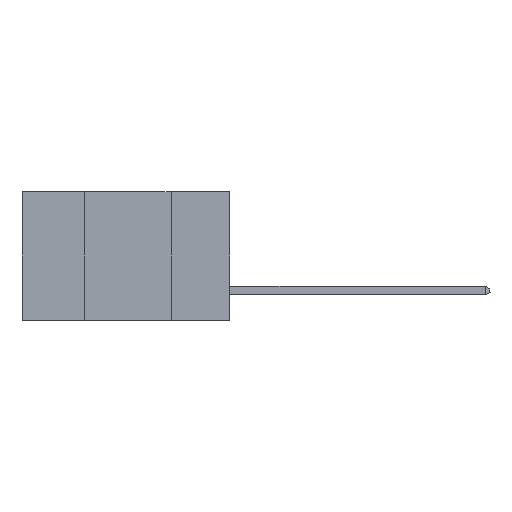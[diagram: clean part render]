
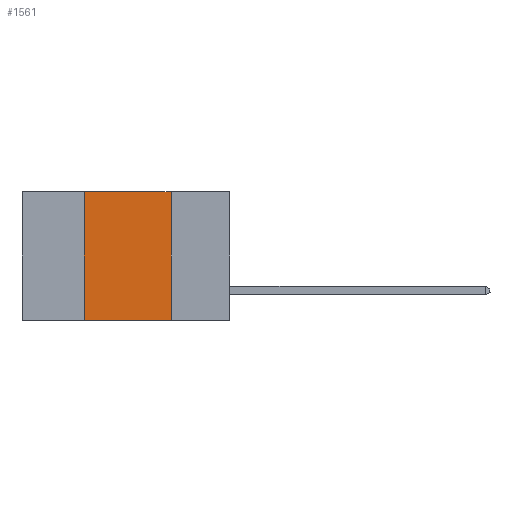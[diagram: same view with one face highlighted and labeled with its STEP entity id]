
A CAD part, left-side view. The second image highlights one B-rep face of the part: STEP entity #1561.
In plain terms, the highlighted planar face has unit normal (-1, 0, 0).
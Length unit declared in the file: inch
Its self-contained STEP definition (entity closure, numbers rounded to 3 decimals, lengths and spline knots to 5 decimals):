
#618 = LINE ( 'NONE', #4870, #1174 ) ;
#1030 = CARTESIAN_POINT ( 'NONE',  ( 0., 0.6, 0. ) ) ;
#1151 = CARTESIAN_POINT ( 'NONE',  ( 0., 0.17, -0.37 ) ) ;
#1174 = VECTOR ( 'NONE', #13529, 39.37008 ) ;
#1247 = DIRECTION ( 'NONE',  ( 1., 0., 0. ) ) ;
#1561 = ADVANCED_FACE ( 'NONE', ( #11752 ), #18600, .F. ) ;
#1626 = DIRECTION ( 'NONE',  ( 0., 0., -1. ) ) ;
#1696 = ORIENTED_EDGE ( 'NONE', *, *, #13982, .F. ) ;
#2046 = VECTOR ( 'NONE', #21828, 39.37008 ) ;
#2376 = DIRECTION ( 'NONE',  ( 0., -1., 0. ) ) ;
#3007 = DIRECTION ( 'NONE',  ( 0., 0., -1. ) ) ;
#4070 = EDGE_CURVE ( 'NONE', #9332, #19464, #14641, .T. ) ;
#4870 = CARTESIAN_POINT ( 'NONE',  ( 0., 0.42, 0. ) ) ;
#5847 = EDGE_LOOP ( 'NONE', ( #14112, #1696, #8938, #15281 ) ) ;
#6528 = CARTESIAN_POINT ( 'NONE',  ( 0., 0.42, 0. ) ) ;
#7306 = AXIS2_PLACEMENT_3D ( 'NONE', #11660, #1247, #3007 ) ;
#7389 = VERTEX_POINT ( 'NONE', #6528 ) ;
#7466 = VECTOR ( 'NONE', #2376, 39.37008 ) ;
#8334 = CARTESIAN_POINT ( 'NONE',  ( 0., 0.17, 0. ) ) ;
#8608 = LINE ( 'NONE', #1030, #2046 ) ;
#8803 = EDGE_CURVE ( 'NONE', #20949, #19464, #17324, .T. ) ;
#8938 = ORIENTED_EDGE ( 'NONE', *, *, #10212, .F. ) ;
#9332 = VERTEX_POINT ( 'NONE', #12645 ) ;
#10212 = EDGE_CURVE ( 'NONE', #20949, #7389, #618, .T. ) ;
#11660 = CARTESIAN_POINT ( 'NONE',  ( 0., 0.6, 0. ) ) ;
#11752 = FACE_OUTER_BOUND ( 'NONE', #5847, .T. ) ;
#12645 = CARTESIAN_POINT ( 'NONE',  ( 0., 0.17, 0. ) ) ;
#13529 = DIRECTION ( 'NONE',  ( 0., 0., 1. ) ) ;
#13982 = EDGE_CURVE ( 'NONE', #7389, #9332, #8608, .T. ) ;
#14112 = ORIENTED_EDGE ( 'NONE', *, *, #4070, .F. ) ;
#14641 = LINE ( 'NONE', #8334, #15201 ) ;
#15201 = VECTOR ( 'NONE', #1626, 39.37008 ) ;
#15281 = ORIENTED_EDGE ( 'NONE', *, *, #8803, .T. ) ;
#17324 = LINE ( 'NONE', #21497, #7466 ) ;
#17548 = CARTESIAN_POINT ( 'NONE',  ( 0., 0.42, -0.37 ) ) ;
#18600 = PLANE ( 'NONE',  #7306 ) ;
#19464 = VERTEX_POINT ( 'NONE', #1151 ) ;
#20949 = VERTEX_POINT ( 'NONE', #17548 ) ;
#21497 = CARTESIAN_POINT ( 'NONE',  ( 0., 0.6, -0.37 ) ) ;
#21828 = DIRECTION ( 'NONE',  ( 0., -1., 0. ) ) ;
